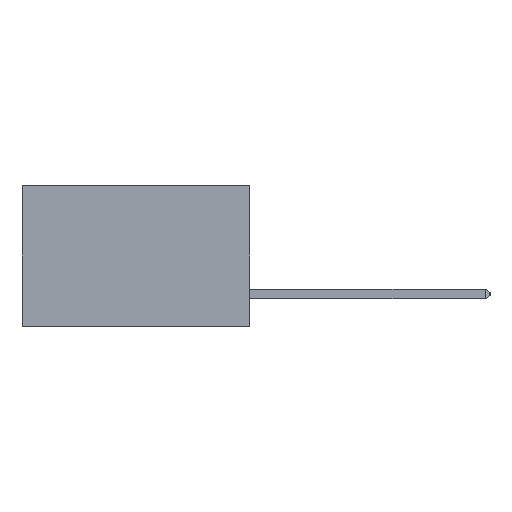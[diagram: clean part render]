
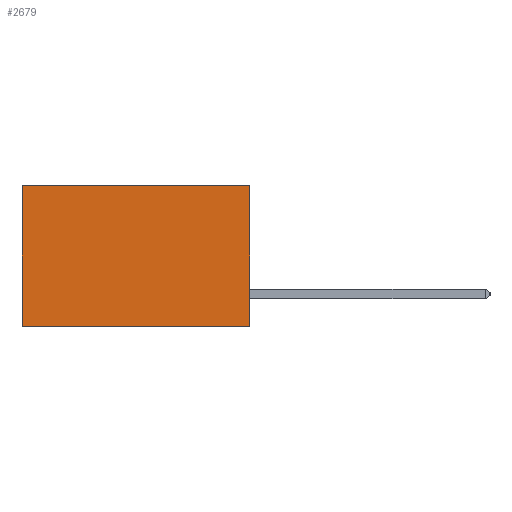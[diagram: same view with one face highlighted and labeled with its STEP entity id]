
A CAD part, left-side view. The second image highlights one B-rep face of the part: STEP entity #2679.
In plain terms, the highlighted planar face has unit normal (-1, 0, 0).
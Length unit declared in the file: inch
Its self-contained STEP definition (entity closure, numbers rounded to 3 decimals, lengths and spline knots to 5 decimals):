
#441 = LINE ( 'NONE', #19892, #16604 ) ;
#630 = FACE_OUTER_BOUND ( 'NONE', #17602, .T. ) ;
#1410 = PLANE ( 'NONE',  #7165 ) ;
#2405 = EDGE_CURVE ( 'NONE', #9970, #16410, #14333, .T. ) ;
#2679 = ADVANCED_FACE ( 'NONE', ( #630 ), #1410, .F. ) ;
#4566 = DIRECTION ( 'NONE',  ( 1., 0., 0. ) ) ;
#4779 = VERTEX_POINT ( 'NONE', #5600 ) ;
#5600 = CARTESIAN_POINT ( 'NONE',  ( 0.2875, 0., 0. ) ) ;
#6084 = VECTOR ( 'NONE', #17861, 39.37008 ) ;
#6356 = ORIENTED_EDGE ( 'NONE', *, *, #12895, .T. ) ;
#6409 = DIRECTION ( 'NONE',  ( 0., 0., -1. ) ) ;
#6452 = EDGE_CURVE ( 'NONE', #4779, #9970, #10739, .T. ) ;
#6511 = CARTESIAN_POINT ( 'NONE',  ( 0.2875, 0., 0. ) ) ;
#6598 = CARTESIAN_POINT ( 'NONE',  ( 0.2875, 0., 0. ) ) ;
#7165 = AXIS2_PLACEMENT_3D ( 'NONE', #9412, #4566, #15463 ) ;
#7323 = CARTESIAN_POINT ( 'NONE',  ( 0.2875, 0., -0.37 ) ) ;
#8057 = DIRECTION ( 'NONE',  ( 0., 1., 0. ) ) ;
#8218 = VERTEX_POINT ( 'NONE', #15969 ) ;
#8724 = LINE ( 'NONE', #6511, #17235 ) ;
#9088 = ORIENTED_EDGE ( 'NONE', *, *, #2405, .F. ) ;
#9412 = CARTESIAN_POINT ( 'NONE',  ( 0.2875, 0., 0. ) ) ;
#9970 = VERTEX_POINT ( 'NONE', #11518 ) ;
#10276 = VECTOR ( 'NONE', #6409, 39.37008 ) ;
#10739 = LINE ( 'NONE', #6598, #10276 ) ;
#11518 = CARTESIAN_POINT ( 'NONE',  ( 0.2875, 0., -0.37 ) ) ;
#11619 = CARTESIAN_POINT ( 'NONE',  ( 0.2875, 0.6, -0.37 ) ) ;
#12247 = ORIENTED_EDGE ( 'NONE', *, *, #14976, .T. ) ;
#12895 = EDGE_CURVE ( 'NONE', #8218, #16410, #441, .T. ) ;
#13673 = DIRECTION ( 'NONE',  ( 0., 0., -1. ) ) ;
#14333 = LINE ( 'NONE', #7323, #6084 ) ;
#14976 = EDGE_CURVE ( 'NONE', #4779, #8218, #8724, .T. ) ;
#15463 = DIRECTION ( 'NONE',  ( 0., 0., -1. ) ) ;
#15969 = CARTESIAN_POINT ( 'NONE',  ( 0.2875, 0.6, 0. ) ) ;
#16410 = VERTEX_POINT ( 'NONE', #11619 ) ;
#16604 = VECTOR ( 'NONE', #13673, 39.37008 ) ;
#17235 = VECTOR ( 'NONE', #8057, 39.37008 ) ;
#17602 = EDGE_LOOP ( 'NONE', ( #6356, #9088, #19306, #12247 ) ) ;
#17861 = DIRECTION ( 'NONE',  ( 0., 1., 0. ) ) ;
#19306 = ORIENTED_EDGE ( 'NONE', *, *, #6452, .F. ) ;
#19892 = CARTESIAN_POINT ( 'NONE',  ( 0.2875, 0.6, 0. ) ) ;
